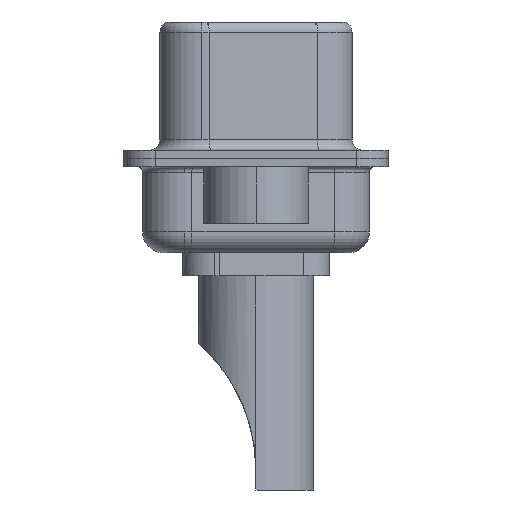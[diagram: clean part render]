
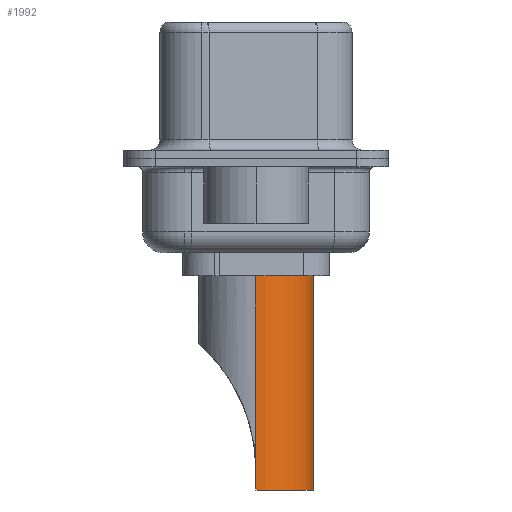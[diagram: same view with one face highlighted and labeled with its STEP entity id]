
A CAD part, left-side view. The second image highlights one B-rep face of the part: STEP entity #1992.
In plain terms, the highlighted cylindrical face has radius 2.75 mm (diameter 5.5 mm), a partial arc.
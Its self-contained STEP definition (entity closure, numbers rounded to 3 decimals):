
#255 = EDGE_CURVE ( 'NONE', #19119, #7129, #19816, .T. ) ;
#364 = EDGE_CURVE ( 'NONE', #23936, #19119, #22597, .T. ) ;
#922 = DIRECTION ( 'NONE',  ( 0., 0., 1. ) ) ;
#941 = CARTESIAN_POINT ( 'NONE',  ( 2.75, 0., -7.764 ) ) ;
#1992 = ADVANCED_FACE ( 'NONE', ( #25053 ), #24439, .T. ) ;
#2555 = AXIS2_PLACEMENT_3D ( 'NONE', #13197, #922, #15247 ) ;
#3254 = LINE ( 'NONE', #26294, #13525 ) ;
#3555 = CARTESIAN_POINT ( 'NONE',  ( -2.75, 0., -8.7 ) ) ;
#4038 = EDGE_LOOP ( 'NONE', ( #18223, #23098, #13514, #14927, #5453, #17899 ) ) ;
#4647 = CARTESIAN_POINT ( 'NONE',  ( 0., 0., 4.234 ) ) ;
#5137 = CARTESIAN_POINT ( 'NONE',  ( 2.75, 0., 4.234 ) ) ;
#5333 = AXIS2_PLACEMENT_3D ( 'NONE', #11459, #17317, #18120 ) ;
#5433 = VERTEX_POINT ( 'NONE', #941 ) ;
#5453 = ORIENTED_EDGE ( 'NONE', *, *, #16340, .T. ) ;
#5648 = VERTEX_POINT ( 'NONE', #19893 ) ;
#5853 = DIRECTION ( 'NONE',  ( 0., 0., -1. ) ) ;
#7129 = VERTEX_POINT ( 'NONE', #19056 ) ;
#8528 = CARTESIAN_POINT ( 'NONE',  ( -2.75, 0., -7.764 ) ) ;
#8783 = VECTOR ( 'NONE', #5853, 1000. ) ;
#9039 = CARTESIAN_POINT ( 'NONE',  ( -2.75, 0., 1.5 ) ) ;
#9874 = EDGE_CURVE ( 'NONE', #22232, #5648, #18934, .T. ) ;
#11244 = LINE ( 'NONE', #5137, #21344 ) ;
#11285 = EDGE_CURVE ( 'NONE', #23936, #22232, #19538, .T. ) ;
#11403 = DIRECTION ( 'NONE',  ( 0., 0., 1. ) ) ;
#11459 = CARTESIAN_POINT ( 'NONE',  ( 0., 0., 1.5 ) ) ;
#11919 = VECTOR ( 'NONE', #12552, 1000. ) ;
#12252 = DIRECTION ( 'NONE',  ( 0., 0., -1. ) ) ;
#12552 = DIRECTION ( 'NONE',  ( 0., 0., 1. ) ) ;
#13197 = CARTESIAN_POINT ( 'NONE',  ( 0., 0., -8.7 ) ) ;
#13514 = ORIENTED_EDGE ( 'NONE', *, *, #9874, .T. ) ;
#13525 = VECTOR ( 'NONE', #12252, 1000. ) ;
#13643 = CARTESIAN_POINT ( 'NONE',  ( -2.75, 0., 4.234 ) ) ;
#14927 = ORIENTED_EDGE ( 'NONE', *, *, #25711, .F. ) ;
#15247 = DIRECTION ( 'NONE',  ( 1., 0., 0. ) ) ;
#16106 = CARTESIAN_POINT ( 'NONE',  ( -2.75, 0., -8.7 ) ) ;
#16340 = EDGE_CURVE ( 'NONE', #5433, #7129, #11244, .T. ) ;
#17317 = DIRECTION ( 'NONE',  ( 0., 0., 1. ) ) ;
#17899 = ORIENTED_EDGE ( 'NONE', *, *, #255, .F. ) ;
#18120 = DIRECTION ( 'NONE',  ( 1., 0., 0. ) ) ;
#18223 = ORIENTED_EDGE ( 'NONE', *, *, #364, .F. ) ;
#18657 = AXIS2_PLACEMENT_3D ( 'NONE', #4647, #24599, #24550 ) ;
#18934 = CIRCLE ( 'NONE', #2555, 2.75 ) ;
#19056 = CARTESIAN_POINT ( 'NONE',  ( 2.75, 0., 1.5 ) ) ;
#19119 = VERTEX_POINT ( 'NONE', #9039 ) ;
#19538 = LINE ( 'NONE', #16106, #8783 ) ;
#19816 = CIRCLE ( 'NONE', #5333, 2.75 ) ;
#19893 = CARTESIAN_POINT ( 'NONE',  ( 2.75, 0., -8.7 ) ) ;
#21344 = VECTOR ( 'NONE', #11403, 1000. ) ;
#22232 = VERTEX_POINT ( 'NONE', #3555 ) ;
#22597 = LINE ( 'NONE', #13643, #11919 ) ;
#23098 = ORIENTED_EDGE ( 'NONE', *, *, #11285, .T. ) ;
#23936 = VERTEX_POINT ( 'NONE', #8528 ) ;
#24439 = CYLINDRICAL_SURFACE ( 'NONE', #18657, 2.75 ) ;
#24550 = DIRECTION ( 'NONE',  ( 1., 0., 0. ) ) ;
#24599 = DIRECTION ( 'NONE',  ( 0., 0., 1. ) ) ;
#25053 = FACE_OUTER_BOUND ( 'NONE', #4038, .T. ) ;
#25711 = EDGE_CURVE ( 'NONE', #5433, #5648, #3254, .T. ) ;
#26294 = CARTESIAN_POINT ( 'NONE',  ( 2.75, 0., -8.7 ) ) ;
